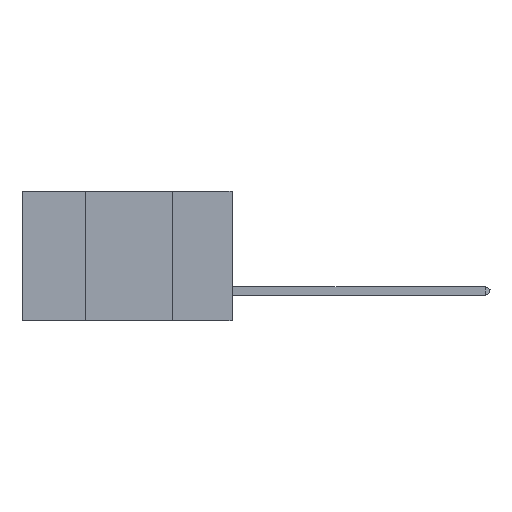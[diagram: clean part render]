
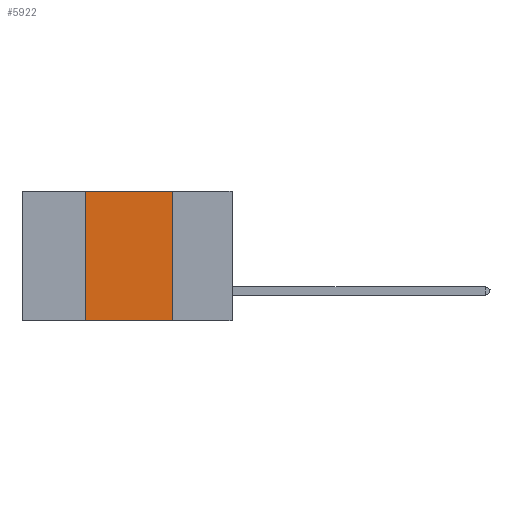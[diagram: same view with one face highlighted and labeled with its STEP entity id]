
A CAD part, left-side view. The second image highlights one B-rep face of the part: STEP entity #5922.
In plain terms, the highlighted planar face has unit normal (-1, 0, 0).
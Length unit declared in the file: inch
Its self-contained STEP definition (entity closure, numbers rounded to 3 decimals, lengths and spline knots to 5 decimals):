
#24 = LINE ( 'NONE', #20391, #36480 ) ;
#876 = DIRECTION ( 'NONE',  ( 0., -1., 0. ) ) ;
#1563 = VECTOR ( 'NONE', #876, 39.37008 ) ;
#2731 = DIRECTION ( 'NONE',  ( 0., -1., 0. ) ) ;
#3264 = DIRECTION ( 'NONE',  ( 1., 0., 0. ) ) ;
#5192 = CARTESIAN_POINT ( 'NONE',  ( 0., 0.17, -0.37 ) ) ;
#5922 = ADVANCED_FACE ( 'NONE', ( #8422 ), #42264, .F. ) ;
#6267 = EDGE_CURVE ( 'NONE', #44544, #36042, #24, .T. ) ;
#6618 = VERTEX_POINT ( 'NONE', #5192 ) ;
#6997 = DIRECTION ( 'NONE',  ( 0., 0., -1. ) ) ;
#7263 = CARTESIAN_POINT ( 'NONE',  ( 0., 0.6, 0. ) ) ;
#8422 = FACE_OUTER_BOUND ( 'NONE', #29550, .T. ) ;
#9909 = LINE ( 'NONE', #22047, #1563 ) ;
#10519 = VECTOR ( 'NONE', #2731, 39.37008 ) ;
#13559 = ORIENTED_EDGE ( 'NONE', *, *, #38997, .F. ) ;
#14131 = ORIENTED_EDGE ( 'NONE', *, *, #20304, .F. ) ;
#14847 = VERTEX_POINT ( 'NONE', #31413 ) ;
#14897 = LINE ( 'NONE', #45015, #10519 ) ;
#18762 = EDGE_CURVE ( 'NONE', #44544, #6618, #14897, .T. ) ;
#20304 = EDGE_CURVE ( 'NONE', #36042, #14847, #9909, .T. ) ;
#20391 = CARTESIAN_POINT ( 'NONE',  ( 0., 0.42, 0. ) ) ;
#22047 = CARTESIAN_POINT ( 'NONE',  ( 0., 0.6, 0. ) ) ;
#23974 = ORIENTED_EDGE ( 'NONE', *, *, #18762, .T. ) ;
#27305 = DIRECTION ( 'NONE',  ( 0., 0., 1. ) ) ;
#29550 = EDGE_LOOP ( 'NONE', ( #13559, #14131, #40016, #23974 ) ) ;
#31413 = CARTESIAN_POINT ( 'NONE',  ( 0., 0.17, 0. ) ) ;
#33452 = AXIS2_PLACEMENT_3D ( 'NONE', #7263, #3264, #35308 ) ;
#34308 = VECTOR ( 'NONE', #6997, 39.37008 ) ;
#34897 = CARTESIAN_POINT ( 'NONE',  ( 0., 0.17, 0. ) ) ;
#35308 = DIRECTION ( 'NONE',  ( 0., 0., -1. ) ) ;
#36042 = VERTEX_POINT ( 'NONE', #38416 ) ;
#36480 = VECTOR ( 'NONE', #27305, 39.37008 ) ;
#38416 = CARTESIAN_POINT ( 'NONE',  ( 0., 0.42, 0. ) ) ;
#38997 = EDGE_CURVE ( 'NONE', #14847, #6618, #40389, .T. ) ;
#40016 = ORIENTED_EDGE ( 'NONE', *, *, #6267, .F. ) ;
#40389 = LINE ( 'NONE', #34897, #34308 ) ;
#42264 = PLANE ( 'NONE',  #33452 ) ;
#42638 = CARTESIAN_POINT ( 'NONE',  ( 0., 0.42, -0.37 ) ) ;
#44544 = VERTEX_POINT ( 'NONE', #42638 ) ;
#45015 = CARTESIAN_POINT ( 'NONE',  ( 0., 0.6, -0.37 ) ) ;
